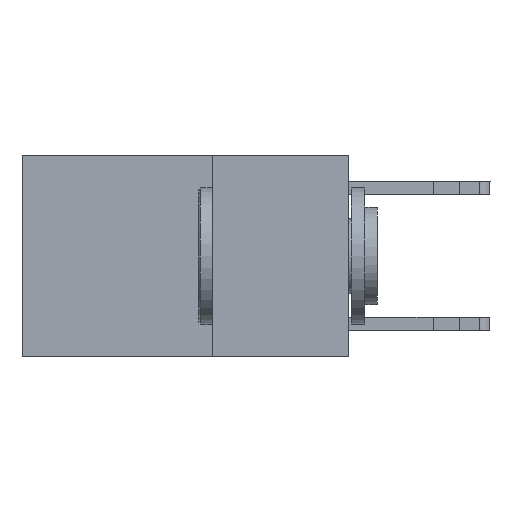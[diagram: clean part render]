
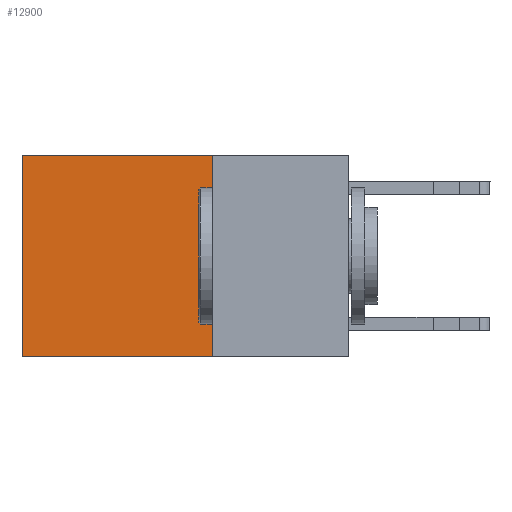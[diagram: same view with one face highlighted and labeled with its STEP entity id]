
A CAD part, left-side view. The second image highlights one B-rep face of the part: STEP entity #12900.
In plain terms, the highlighted planar face has unit normal (-1, 0, 0).
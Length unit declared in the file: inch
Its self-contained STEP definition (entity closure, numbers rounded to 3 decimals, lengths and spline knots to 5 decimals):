
#1721 = CARTESIAN_POINT ( 'NONE',  ( 0.2625, 0.6, 0. ) ) ;
#1819 = LINE ( 'NONE', #6390, #11462 ) ;
#2055 = CARTESIAN_POINT ( 'NONE',  ( 0.2625, 0.25, 0. ) ) ;
#4216 = EDGE_CURVE ( 'NONE', #22929, #20552, #1819, .T. ) ;
#5113 = CARTESIAN_POINT ( 'NONE',  ( 0.2625, 0.6, 0. ) ) ;
#5512 = LINE ( 'NONE', #1721, #8717 ) ;
#6390 = CARTESIAN_POINT ( 'NONE',  ( 0.2625, 0.25, 0. ) ) ;
#6710 = VECTOR ( 'NONE', #23015, 39.37008 ) ;
#7571 = ORIENTED_EDGE ( 'NONE', *, *, #10146, .F. ) ;
#8717 = VECTOR ( 'NONE', #15991, 39.37008 ) ;
#9921 = PLANE ( 'NONE',  #21299 ) ;
#10146 = EDGE_CURVE ( 'NONE', #22929, #11803, #19025, .T. ) ;
#11462 = VECTOR ( 'NONE', #14399, 39.37008 ) ;
#11803 = VERTEX_POINT ( 'NONE', #21643 ) ;
#12478 = VECTOR ( 'NONE', #22698, 39.37008 ) ;
#12499 = ORIENTED_EDGE ( 'NONE', *, *, #23459, .T. ) ;
#12900 = ADVANCED_FACE ( 'NONE', ( #13978 ), #9921, .F. ) ;
#13082 = CARTESIAN_POINT ( 'NONE',  ( 0.2625, 0.25, -0.37 ) ) ;
#13323 = CARTESIAN_POINT ( 'NONE',  ( 0.2625, 0.25, 0. ) ) ;
#13978 = FACE_OUTER_BOUND ( 'NONE', #17692, .T. ) ;
#14399 = DIRECTION ( 'NONE',  ( 0., 1., 0. ) ) ;
#14865 = EDGE_CURVE ( 'NONE', #11803, #20242, #15283, .T. ) ;
#15011 = ORIENTED_EDGE ( 'NONE', *, *, #4216, .T. ) ;
#15283 = LINE ( 'NONE', #13082, #6710 ) ;
#15363 = CARTESIAN_POINT ( 'NONE',  ( 0.2625, 0.6, -0.37 ) ) ;
#15991 = DIRECTION ( 'NONE',  ( 0., 0., -1. ) ) ;
#17692 = EDGE_LOOP ( 'NONE', ( #12499, #19022, #7571, #15011 ) ) ;
#18940 = DIRECTION ( 'NONE',  ( 1., 0., 0. ) ) ;
#19022 = ORIENTED_EDGE ( 'NONE', *, *, #14865, .F. ) ;
#19025 = LINE ( 'NONE', #25157, #12478 ) ;
#20242 = VERTEX_POINT ( 'NONE', #15363 ) ;
#20552 = VERTEX_POINT ( 'NONE', #5113 ) ;
#21299 = AXIS2_PLACEMENT_3D ( 'NONE', #2055, #18940, #24437 ) ;
#21643 = CARTESIAN_POINT ( 'NONE',  ( 0.2625, 0.25, -0.37 ) ) ;
#22698 = DIRECTION ( 'NONE',  ( 0., 0., -1. ) ) ;
#22929 = VERTEX_POINT ( 'NONE', #13323 ) ;
#23015 = DIRECTION ( 'NONE',  ( 0., 1., 0. ) ) ;
#23459 = EDGE_CURVE ( 'NONE', #20552, #20242, #5512, .T. ) ;
#24437 = DIRECTION ( 'NONE',  ( 0., 0., -1. ) ) ;
#25157 = CARTESIAN_POINT ( 'NONE',  ( 0.2625, 0.25, 0. ) ) ;
